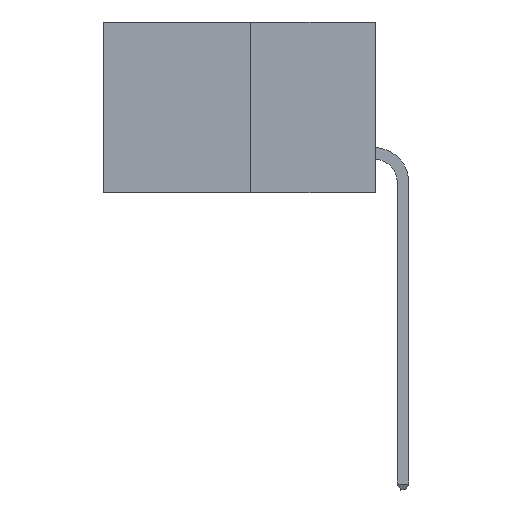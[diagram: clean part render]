
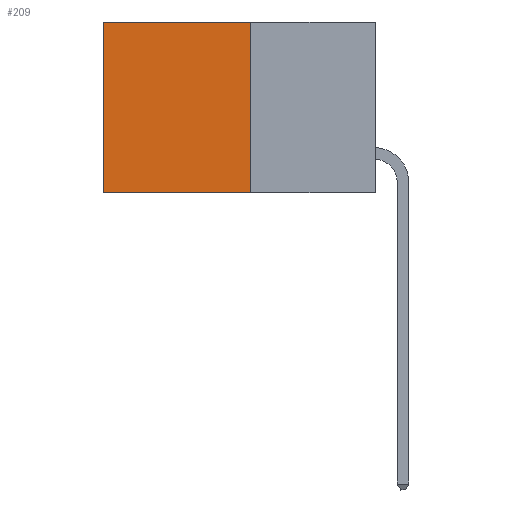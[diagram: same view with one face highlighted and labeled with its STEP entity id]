
A CAD part, left-side view. The second image highlights one B-rep face of the part: STEP entity #209.
In plain terms, the highlighted planar face has unit normal (-1, 0, 0).
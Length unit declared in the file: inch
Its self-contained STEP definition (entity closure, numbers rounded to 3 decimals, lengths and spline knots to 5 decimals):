
#176 = AXIS2_PLACEMENT_3D ( 'NONE', #2700, #5366, #638 ) ;
#209 = ADVANCED_FACE ( 'NONE', ( #229 ), #310, .F. ) ;
#229 = FACE_OUTER_BOUND ( 'NONE', #4993, .T. ) ;
#310 = PLANE ( 'NONE',  #176 ) ;
#537 = VECTOR ( 'NONE', #8467, 39.37008 ) ;
#638 = DIRECTION ( 'NONE',  ( 0., 0., -1. ) ) ;
#771 = LINE ( 'NONE', #4506, #537 ) ;
#1173 = DIRECTION ( 'NONE',  ( 0., 0., -1. ) ) ;
#1298 = EDGE_CURVE ( 'NONE', #8828, #1667, #771, .T. ) ;
#1571 = ORIENTED_EDGE ( 'NONE', *, *, #7188, .F. ) ;
#1667 = VERTEX_POINT ( 'NONE', #1803 ) ;
#1803 = CARTESIAN_POINT ( 'NONE',  ( 0.277, 0.59, -0.37 ) ) ;
#2127 = LINE ( 'NONE', #2149, #7757 ) ;
#2149 = CARTESIAN_POINT ( 'NONE',  ( 0.277, 0.27, 0. ) ) ;
#2700 = CARTESIAN_POINT ( 'NONE',  ( 0.277, 0.27, -0.37 ) ) ;
#3072 = EDGE_CURVE ( 'NONE', #3358, #5152, #2127, .T. ) ;
#3305 = ORIENTED_EDGE ( 'NONE', *, *, #8558, .T. ) ;
#3358 = VERTEX_POINT ( 'NONE', #5123 ) ;
#3710 = LINE ( 'NONE', #4372, #7391 ) ;
#3751 = DIRECTION ( 'NONE',  ( 0., 0., -1. ) ) ;
#4372 = CARTESIAN_POINT ( 'NONE',  ( 0.277, 0.59, -0.37 ) ) ;
#4506 = CARTESIAN_POINT ( 'NONE',  ( 0.277, 0.27, -0.37 ) ) ;
#4840 = VECTOR ( 'NONE', #1173, 39.37008 ) ;
#4993 = EDGE_LOOP ( 'NONE', ( #3305, #7037, #1571, #5396 ) ) ;
#5123 = CARTESIAN_POINT ( 'NONE',  ( 0.277, 0.27, 0. ) ) ;
#5152 = VERTEX_POINT ( 'NONE', #7064 ) ;
#5366 = DIRECTION ( 'NONE',  ( 1., 0., 0. ) ) ;
#5396 = ORIENTED_EDGE ( 'NONE', *, *, #3072, .T. ) ;
#7037 = ORIENTED_EDGE ( 'NONE', *, *, #1298, .F. ) ;
#7064 = CARTESIAN_POINT ( 'NONE',  ( 0.277, 0.59, 0. ) ) ;
#7188 = EDGE_CURVE ( 'NONE', #3358, #8828, #7527, .T. ) ;
#7391 = VECTOR ( 'NONE', #3751, 39.37008 ) ;
#7477 = DIRECTION ( 'NONE',  ( 0., 1., 0. ) ) ;
#7527 = LINE ( 'NONE', #8539, #4840 ) ;
#7757 = VECTOR ( 'NONE', #7477, 39.37008 ) ;
#8467 = DIRECTION ( 'NONE',  ( 0., 1., 0. ) ) ;
#8539 = CARTESIAN_POINT ( 'NONE',  ( 0.277, 0.27, -0.37 ) ) ;
#8558 = EDGE_CURVE ( 'NONE', #5152, #1667, #3710, .T. ) ;
#8828 = VERTEX_POINT ( 'NONE', #8959 ) ;
#8959 = CARTESIAN_POINT ( 'NONE',  ( 0.277, 0.27, -0.37 ) ) ;
